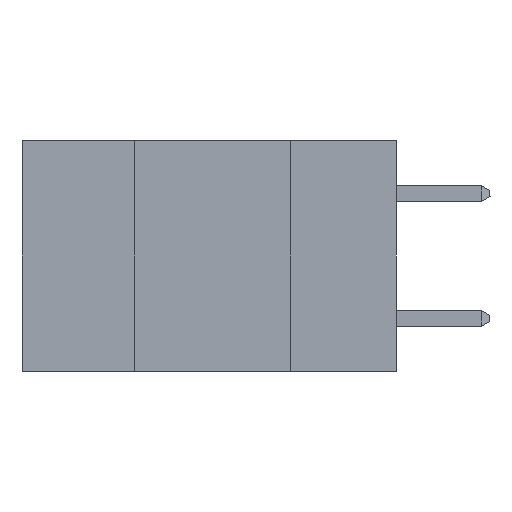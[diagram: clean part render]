
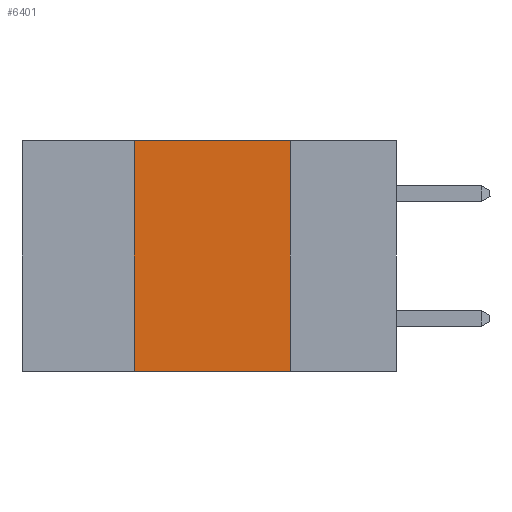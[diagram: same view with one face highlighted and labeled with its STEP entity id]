
A CAD part, left-side view. The second image highlights one B-rep face of the part: STEP entity #6401.
In plain terms, the highlighted planar face has unit normal (-1, 0, 0).
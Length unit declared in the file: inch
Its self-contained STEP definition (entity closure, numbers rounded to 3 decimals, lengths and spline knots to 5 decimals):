
#2352 = VECTOR ( 'NONE', #9167, 39.37008 ) ;
#2674 = CARTESIAN_POINT ( 'NONE',  ( 0., 0.17, -0.37 ) ) ;
#3177 = CARTESIAN_POINT ( 'NONE',  ( 0., 0.17, 0. ) ) ;
#3623 = AXIS2_PLACEMENT_3D ( 'NONE', #4585, #19235, #6573 ) ;
#4585 = CARTESIAN_POINT ( 'NONE',  ( 0., 0.6, 0. ) ) ;
#4784 = FACE_OUTER_BOUND ( 'NONE', #16406, .T. ) ;
#5210 = VERTEX_POINT ( 'NONE', #12370 ) ;
#5558 = VERTEX_POINT ( 'NONE', #19200 ) ;
#5977 = VECTOR ( 'NONE', #17490, 39.37008 ) ;
#6401 = ADVANCED_FACE ( 'NONE', ( #4784 ), #10072, .F. ) ;
#6573 = DIRECTION ( 'NONE',  ( 0., 0., -1. ) ) ;
#6832 = LINE ( 'NONE', #3177, #5977 ) ;
#8837 = CARTESIAN_POINT ( 'NONE',  ( 0., 0.42, 0. ) ) ;
#9153 = VECTOR ( 'NONE', #21939, 39.37008 ) ;
#9167 = DIRECTION ( 'NONE',  ( 0., 0., 1. ) ) ;
#9974 = CARTESIAN_POINT ( 'NONE',  ( 0., 0.6, -0.37 ) ) ;
#10072 = PLANE ( 'NONE',  #3623 ) ;
#11729 = DIRECTION ( 'NONE',  ( 0., -1., 0. ) ) ;
#12370 = CARTESIAN_POINT ( 'NONE',  ( 0., 0.42, -0.37 ) ) ;
#13446 = LINE ( 'NONE', #18106, #9153 ) ;
#13593 = EDGE_CURVE ( 'NONE', #19378, #5558, #13446, .T. ) ;
#15179 = VECTOR ( 'NONE', #11729, 39.37008 ) ;
#16406 = EDGE_LOOP ( 'NONE', ( #23222, #21318, #19057, #21816 ) ) ;
#17154 = EDGE_CURVE ( 'NONE', #5210, #19378, #22601, .T. ) ;
#17490 = DIRECTION ( 'NONE',  ( 0., 0., -1. ) ) ;
#18106 = CARTESIAN_POINT ( 'NONE',  ( 0., 0.6, 0. ) ) ;
#18263 = CARTESIAN_POINT ( 'NONE',  ( 0., 0.42, 0. ) ) ;
#18680 = VERTEX_POINT ( 'NONE', #2674 ) ;
#18974 = EDGE_CURVE ( 'NONE', #5558, #18680, #6832, .T. ) ;
#19057 = ORIENTED_EDGE ( 'NONE', *, *, #17154, .F. ) ;
#19200 = CARTESIAN_POINT ( 'NONE',  ( 0., 0.17, 0. ) ) ;
#19235 = DIRECTION ( 'NONE',  ( 1., 0., 0. ) ) ;
#19378 = VERTEX_POINT ( 'NONE', #8837 ) ;
#20051 = LINE ( 'NONE', #9974, #15179 ) ;
#21318 = ORIENTED_EDGE ( 'NONE', *, *, #13593, .F. ) ;
#21816 = ORIENTED_EDGE ( 'NONE', *, *, #23015, .T. ) ;
#21939 = DIRECTION ( 'NONE',  ( 0., -1., 0. ) ) ;
#22601 = LINE ( 'NONE', #18263, #2352 ) ;
#23015 = EDGE_CURVE ( 'NONE', #5210, #18680, #20051, .T. ) ;
#23222 = ORIENTED_EDGE ( 'NONE', *, *, #18974, .F. ) ;
